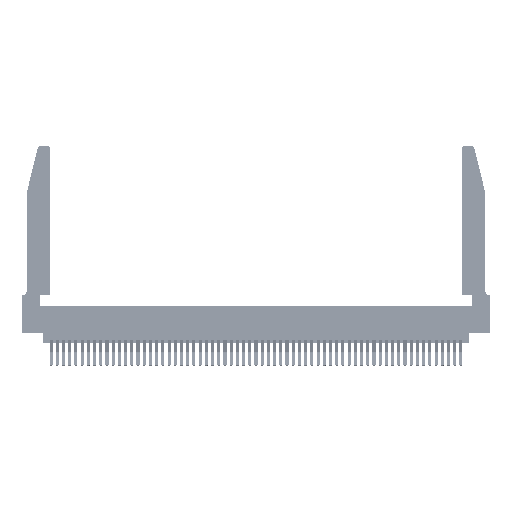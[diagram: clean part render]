
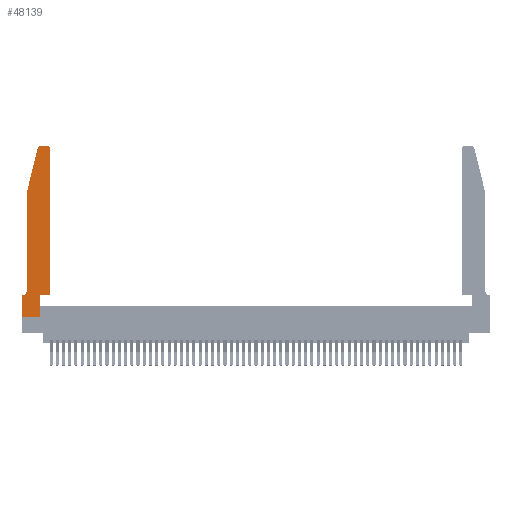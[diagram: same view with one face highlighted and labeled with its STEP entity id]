
A CAD part, top view. The second image highlights one B-rep face of the part: STEP entity #48139.
In plain terms, the highlighted planar face has unit normal (0, 0, 1).
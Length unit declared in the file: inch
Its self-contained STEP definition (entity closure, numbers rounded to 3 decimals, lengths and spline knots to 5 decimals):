
#4 = VERTEX_POINT ( 'NONE', #23254 ) ;
#32 = CARTESIAN_POINT ( 'NONE',  ( 0.25487, 2.72718, 0.37 ) ) ;
#392 = ORIENTED_EDGE ( 'NONE', *, *, #14781, .T. ) ;
#659 = DIRECTION ( 'NONE',  ( 0., -1., 0. ) ) ;
#838 = EDGE_LOOP ( 'NONE', ( #9757, #9939, #42203, #42808, #392, #38377, #7036, #46936, #3847, #23985, #21937, #19990 ) ) ;
#1022 = EDGE_CURVE ( 'NONE', #32336, #47264, #35971, .T. ) ;
#2031 = CARTESIAN_POINT ( 'NONE',  ( 0.0755, 2., 0.37 ) ) ;
#2285 = EDGE_CURVE ( 'NONE', #3389, #14889, #30013, .T. ) ;
#3051 = DIRECTION ( 'NONE',  ( 0., 0., 1. ) ) ;
#3389 = VERTEX_POINT ( 'NONE', #32824 ) ;
#3847 = ORIENTED_EDGE ( 'NONE', *, *, #30887, .T. ) ;
#4032 = CARTESIAN_POINT ( 'NONE',  ( 0.284, 2.72, 0.37 ) ) ;
#4233 = VERTEX_POINT ( 'NONE', #45451 ) ;
#5170 = VERTEX_POINT ( 'NONE', #34208 ) ;
#5580 = CARTESIAN_POINT ( 'NONE',  ( 0.4505, 2.72, 0.37 ) ) ;
#5873 = DIRECTION ( 'NONE',  ( -1., 0., 0. ) ) ;
#6463 = CIRCLE ( 'NONE', #42445, 0.03 ) ;
#6554 = EDGE_CURVE ( 'NONE', #52166, #3389, #37703, .T. ) ;
#7036 = ORIENTED_EDGE ( 'NONE', *, *, #1022, .T. ) ;
#7367 = VECTOR ( 'NONE', #10785, 39.37008 ) ;
#7720 = DIRECTION ( 'NONE',  ( 0., 0., 1. ) ) ;
#8527 = EDGE_CURVE ( 'NONE', #47264, #20587, #41412, .T. ) ;
#9009 = EDGE_CURVE ( 'NONE', #15211, #14821, #34829, .T. ) ;
#9757 = ORIENTED_EDGE ( 'NONE', *, *, #18578, .T. ) ;
#9939 = ORIENTED_EDGE ( 'NONE', *, *, #50587, .T. ) ;
#10102 = EDGE_CURVE ( 'NONE', #4, #32336, #48009, .T. ) ;
#10298 = CARTESIAN_POINT ( 'NONE',  ( 0.0755, 2., 0.37 ) ) ;
#10785 = DIRECTION ( 'NONE',  ( -0.239, -0.971, 0. ) ) ;
#12015 = LINE ( 'NONE', #10298, #51949 ) ;
#12262 = DIRECTION ( 'NONE',  ( 1., 0., 0. ) ) ;
#14455 = CARTESIAN_POINT ( 'NONE',  ( 0., 0., 0.37 ) ) ;
#14523 = DIRECTION ( 'NONE',  ( 1., 0., 0. ) ) ;
#14639 = CARTESIAN_POINT ( 'NONE',  ( 0.2605, 2.75, 0.37 ) ) ;
#14781 = EDGE_CURVE ( 'NONE', #4233, #4, #51635, .T. ) ;
#14821 = VERTEX_POINT ( 'NONE', #47414 ) ;
#14889 = VERTEX_POINT ( 'NONE', #5580 ) ;
#15087 = EDGE_CURVE ( 'NONE', #14889, #44788, #6463, .T. ) ;
#15211 = VERTEX_POINT ( 'NONE', #32 ) ;
#15227 = DIRECTION ( 'NONE',  ( 1., 0., 0. ) ) ;
#15462 = CARTESIAN_POINT ( 'NONE',  ( 0., 0.35, 0.37 ) ) ;
#16102 = CARTESIAN_POINT ( 'NONE',  ( 0.4205, 2.72, 0.37 ) ) ;
#17384 = CARTESIAN_POINT ( 'NONE',  ( 0., 0.35, 0.37 ) ) ;
#17746 = CARTESIAN_POINT ( 'NONE',  ( 0.2865, 0.35, 0.37 ) ) ;
#18578 = EDGE_CURVE ( 'NONE', #44788, #5170, #28638, .T. ) ;
#19990 = ORIENTED_EDGE ( 'NONE', *, *, #15087, .T. ) ;
#20587 = VERTEX_POINT ( 'NONE', #30785 ) ;
#20775 = FACE_OUTER_BOUND ( 'NONE', #838, .T. ) ;
#21937 = ORIENTED_EDGE ( 'NONE', *, *, #2285, .T. ) ;
#23254 = CARTESIAN_POINT ( 'NONE',  ( 0.0055, 0.35, 0.37 ) ) ;
#23985 = ORIENTED_EDGE ( 'NONE', *, *, #6554, .T. ) ;
#25330 = VECTOR ( 'NONE', #35654, 39.37008 ) ;
#26949 = CARTESIAN_POINT ( 'NONE',  ( 0.4205, 2.75, 0.37 ) ) ;
#27786 = AXIS2_PLACEMENT_3D ( 'NONE', #4032, #41518, #12262 ) ;
#28584 = DIRECTION ( 'NONE',  ( 1., 0., 0. ) ) ;
#28638 = LINE ( 'NONE', #14639, #25330 ) ;
#30013 = LINE ( 'NONE', #35899, #48308 ) ;
#30785 = CARTESIAN_POINT ( 'NONE',  ( 0.2865, 0., 0.37 ) ) ;
#30887 = EDGE_CURVE ( 'NONE', #20587, #52166, #31701, .T. ) ;
#31337 = DIRECTION ( 'NONE',  ( 0., -1., 0. ) ) ;
#31701 = LINE ( 'NONE', #43736, #48636 ) ;
#32336 = VERTEX_POINT ( 'NONE', #17384 ) ;
#32824 = CARTESIAN_POINT ( 'NONE',  ( 0.4505, 0.35, 0.37 ) ) ;
#34208 = CARTESIAN_POINT ( 'NONE',  ( 0.284, 2.75, 0.37 ) ) ;
#34255 = VECTOR ( 'NONE', #5873, 39.37008 ) ;
#34375 = CARTESIAN_POINT ( 'NONE',  ( 0.0755, 0.35, 0.37 ) ) ;
#34829 = LINE ( 'NONE', #2031, #7367 ) ;
#35072 = VECTOR ( 'NONE', #14523, 39.37008 ) ;
#35654 = DIRECTION ( 'NONE',  ( -1., 0., 0. ) ) ;
#35895 = CARTESIAN_POINT ( 'NONE',  ( 0.4505, 0.35, 0.37 ) ) ;
#35899 = CARTESIAN_POINT ( 'NONE',  ( 0.4505, 0.35, 0.37 ) ) ;
#35971 = LINE ( 'NONE', #41805, #37976 ) ;
#36054 = CARTESIAN_POINT ( 'NONE',  ( 0., 0., 0.37 ) ) ;
#36083 = AXIS2_PLACEMENT_3D ( 'NONE', #47053, #37930, #46523 ) ;
#36480 = DIRECTION ( 'NONE',  ( 1., 0., 0. ) ) ;
#37703 = LINE ( 'NONE', #35895, #35072 ) ;
#37930 = DIRECTION ( 'NONE',  ( 0., 0., -1. ) ) ;
#37976 = VECTOR ( 'NONE', #659, 39.37008 ) ;
#38377 = ORIENTED_EDGE ( 'NONE', *, *, #10102, .T. ) ;
#39909 = AXIS2_PLACEMENT_3D ( 'NONE', #15462, #3051, #36480 ) ;
#40512 = PLANE ( 'NONE',  #39909 ) ;
#41412 = LINE ( 'NONE', #36054, #46635 ) ;
#41518 = DIRECTION ( 'NONE',  ( 0., 0., 1. ) ) ;
#41805 = CARTESIAN_POINT ( 'NONE',  ( 0., 0., 0.37 ) ) ;
#42203 = ORIENTED_EDGE ( 'NONE', *, *, #9009, .T. ) ;
#42445 = AXIS2_PLACEMENT_3D ( 'NONE', #16102, #7720, #28584 ) ;
#42808 = ORIENTED_EDGE ( 'NONE', *, *, #44706, .T. ) ;
#43736 = CARTESIAN_POINT ( 'NONE',  ( 0.2865, 0.35, 0.37 ) ) ;
#44706 = EDGE_CURVE ( 'NONE', #14821, #4233, #12015, .T. ) ;
#44788 = VERTEX_POINT ( 'NONE', #26949 ) ;
#45026 = DIRECTION ( 'NONE',  ( 0., 1., 0. ) ) ;
#45451 = CARTESIAN_POINT ( 'NONE',  ( 0.0755, 0.42, 0.37 ) ) ;
#46523 = DIRECTION ( 'NONE',  ( -1., 0., 0. ) ) ;
#46635 = VECTOR ( 'NONE', #15227, 39.37008 ) ;
#46909 = CIRCLE ( 'NONE', #27786, 0.03 ) ;
#46936 = ORIENTED_EDGE ( 'NONE', *, *, #8527, .T. ) ;
#47053 = CARTESIAN_POINT ( 'NONE',  ( 0.0055, 0.42, 0.37 ) ) ;
#47216 = DIRECTION ( 'NONE',  ( 0., 1., 0. ) ) ;
#47264 = VERTEX_POINT ( 'NONE', #14455 ) ;
#47414 = CARTESIAN_POINT ( 'NONE',  ( 0.0755, 2., 0.37 ) ) ;
#48009 = LINE ( 'NONE', #34375, #34255 ) ;
#48139 = ADVANCED_FACE ( 'NONE', ( #20775 ), #40512, .T. ) ;
#48308 = VECTOR ( 'NONE', #45026, 39.37008 ) ;
#48636 = VECTOR ( 'NONE', #47216, 39.37008 ) ;
#50587 = EDGE_CURVE ( 'NONE', #5170, #15211, #46909, .T. ) ;
#51635 = CIRCLE ( 'NONE', #36083, 0.07 ) ;
#51949 = VECTOR ( 'NONE', #31337, 39.37008 ) ;
#52166 = VERTEX_POINT ( 'NONE', #17746 ) ;
